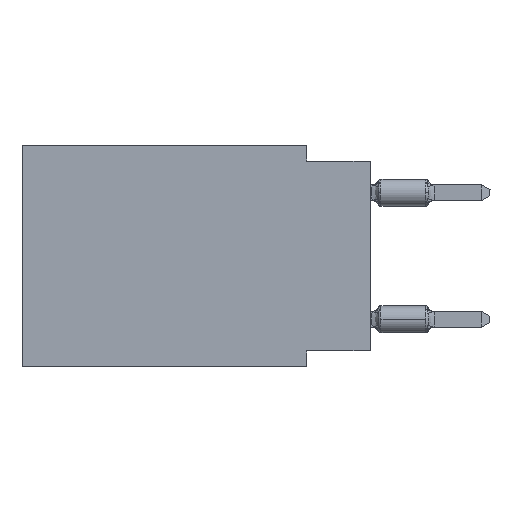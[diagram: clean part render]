
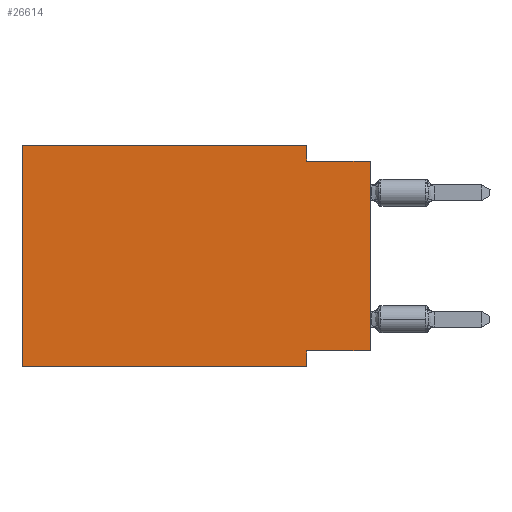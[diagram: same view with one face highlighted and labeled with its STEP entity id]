
A CAD part, left-side view. The second image highlights one B-rep face of the part: STEP entity #26614.
In plain terms, the highlighted planar face has unit normal (-1, 0, 0).
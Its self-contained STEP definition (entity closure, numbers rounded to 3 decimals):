
#291 = DIRECTION ( 'NONE',  ( 0., -1., 0. ) ) ;
#984 = DIRECTION ( 'NONE',  ( 0., 0., -1. ) ) ;
#1086 = EDGE_CURVE ( 'NONE', #29722, #15440, #27906, .T. ) ;
#1136 = DIRECTION ( 'NONE',  ( 0., 0., 1. ) ) ;
#1277 = CARTESIAN_POINT ( 'NONE',  ( 0., 0., 0. ) ) ;
#2271 = CARTESIAN_POINT ( 'NONE',  ( 0., 2.54, 0. ) ) ;
#2378 = LINE ( 'NONE', #13637, #22519 ) ;
#3339 = VECTOR ( 'NONE', #25569, 1000. ) ;
#3637 = LINE ( 'NONE', #1277, #3722 ) ;
#3722 = VECTOR ( 'NONE', #1136, 1000. ) ;
#3803 = EDGE_CURVE ( 'NONE', #14865, #9660, #3637, .T. ) ;
#4396 = CARTESIAN_POINT ( 'NONE',  ( 0., 2.54, -0.635 ) ) ;
#4958 = VECTOR ( 'NONE', #291, 1000. ) ;
#6455 = CARTESIAN_POINT ( 'NONE',  ( 0., 13.97, 0. ) ) ;
#7423 = VECTOR ( 'NONE', #29323, 1000. ) ;
#7798 = CARTESIAN_POINT ( 'NONE',  ( 0., 13.97, 0. ) ) ;
#7844 = ORIENTED_EDGE ( 'NONE', *, *, #26591, .F. ) ;
#8154 = VECTOR ( 'NONE', #13016, 1000. ) ;
#8409 = LINE ( 'NONE', #7798, #14413 ) ;
#9228 = CARTESIAN_POINT ( 'NONE',  ( 0., 2.54, 0. ) ) ;
#9465 = EDGE_CURVE ( 'NONE', #18776, #28046, #16870, .T. ) ;
#9616 = LINE ( 'NONE', #2271, #26015 ) ;
#9660 = VERTEX_POINT ( 'NONE', #25166 ) ;
#10150 = AXIS2_PLACEMENT_3D ( 'NONE', #27435, #27589, #984 ) ;
#10350 = CARTESIAN_POINT ( 'NONE',  ( 0., 2.54, -8.89 ) ) ;
#10510 = ORIENTED_EDGE ( 'NONE', *, *, #16415, .F. ) ;
#10780 = EDGE_CURVE ( 'NONE', #18776, #29722, #8409, .T. ) ;
#10806 = PLANE ( 'NONE',  #10150 ) ;
#11121 = CARTESIAN_POINT ( 'NONE',  ( 0., 0., -8.255 ) ) ;
#11729 = ORIENTED_EDGE ( 'NONE', *, *, #1086, .F. ) ;
#13016 = DIRECTION ( 'NONE',  ( 0., 0., -1. ) ) ;
#13373 = ORIENTED_EDGE ( 'NONE', *, *, #14781, .F. ) ;
#13637 = CARTESIAN_POINT ( 'NONE',  ( 0., 0., -0.635 ) ) ;
#14413 = VECTOR ( 'NONE', #20010, 1000. ) ;
#14481 = VERTEX_POINT ( 'NONE', #22772 ) ;
#14633 = CARTESIAN_POINT ( 'NONE',  ( 0., 13.97, 0. ) ) ;
#14781 = EDGE_CURVE ( 'NONE', #14865, #14481, #22431, .T. ) ;
#14865 = VERTEX_POINT ( 'NONE', #11121 ) ;
#15440 = VERTEX_POINT ( 'NONE', #9228 ) ;
#16415 = EDGE_CURVE ( 'NONE', #15440, #18394, #9616, .T. ) ;
#16817 = EDGE_CURVE ( 'NONE', #18394, #9660, #2378, .T. ) ;
#16870 = LINE ( 'NONE', #18921, #4958 ) ;
#17401 = ORIENTED_EDGE ( 'NONE', *, *, #16817, .F. ) ;
#17862 = FACE_OUTER_BOUND ( 'NONE', #29118, .T. ) ;
#18394 = VERTEX_POINT ( 'NONE', #4396 ) ;
#18776 = VERTEX_POINT ( 'NONE', #26553 ) ;
#18921 = CARTESIAN_POINT ( 'NONE',  ( 0., 13.97, -8.89 ) ) ;
#20010 = DIRECTION ( 'NONE',  ( 0., 0., 1. ) ) ;
#22427 = LINE ( 'NONE', #10350, #8154 ) ;
#22431 = LINE ( 'NONE', #24473, #7423 ) ;
#22519 = VECTOR ( 'NONE', #26053, 1000. ) ;
#22772 = CARTESIAN_POINT ( 'NONE',  ( 0., 2.54, -8.255 ) ) ;
#23462 = ORIENTED_EDGE ( 'NONE', *, *, #3803, .T. ) ;
#24473 = CARTESIAN_POINT ( 'NONE',  ( 0., 0., -8.255 ) ) ;
#25166 = CARTESIAN_POINT ( 'NONE',  ( 0., 0., -0.635 ) ) ;
#25569 = DIRECTION ( 'NONE',  ( 0., -1., 0. ) ) ;
#26015 = VECTOR ( 'NONE', #30937, 1000. ) ;
#26053 = DIRECTION ( 'NONE',  ( 0., -1., 0. ) ) ;
#26553 = CARTESIAN_POINT ( 'NONE',  ( 0., 13.97, -8.89 ) ) ;
#26591 = EDGE_CURVE ( 'NONE', #14481, #28046, #22427, .T. ) ;
#26614 = ADVANCED_FACE ( 'NONE', ( #17862 ), #10806, .F. ) ;
#26764 = ORIENTED_EDGE ( 'NONE', *, *, #9465, .T. ) ;
#27435 = CARTESIAN_POINT ( 'NONE',  ( 0., 13.97, 0. ) ) ;
#27589 = DIRECTION ( 'NONE',  ( 1., 0., 0. ) ) ;
#27874 = ORIENTED_EDGE ( 'NONE', *, *, #10780, .F. ) ;
#27906 = LINE ( 'NONE', #6455, #3339 ) ;
#28046 = VERTEX_POINT ( 'NONE', #29394 ) ;
#29118 = EDGE_LOOP ( 'NONE', ( #23462, #17401, #10510, #11729, #27874, #26764, #7844, #13373 ) ) ;
#29323 = DIRECTION ( 'NONE',  ( 0., 1., 0. ) ) ;
#29394 = CARTESIAN_POINT ( 'NONE',  ( 0., 2.54, -8.89 ) ) ;
#29722 = VERTEX_POINT ( 'NONE', #14633 ) ;
#30937 = DIRECTION ( 'NONE',  ( 0., 0., -1. ) ) ;
